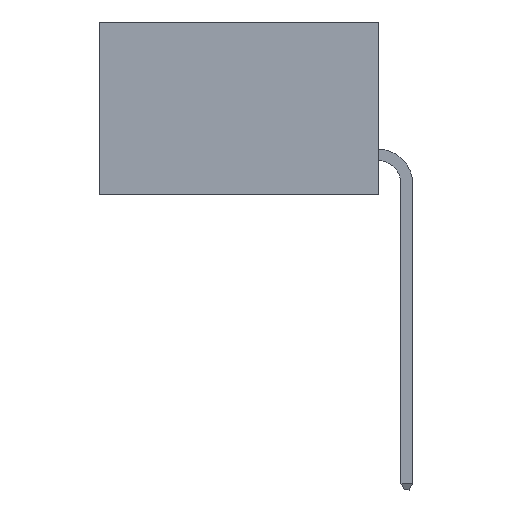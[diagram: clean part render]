
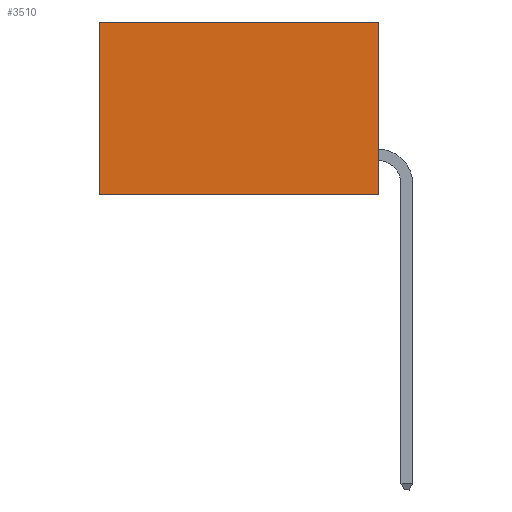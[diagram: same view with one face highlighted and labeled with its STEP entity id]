
A CAD part, left-side view. The second image highlights one B-rep face of the part: STEP entity #3510.
In plain terms, the highlighted planar face has unit normal (-1, 0, 0).
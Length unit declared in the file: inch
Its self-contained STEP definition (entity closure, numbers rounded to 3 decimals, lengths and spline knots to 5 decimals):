
#784 = LINE ( 'NONE', #14270, #11779 ) ;
#1251 = VERTEX_POINT ( 'NONE', #3374 ) ;
#1841 = CARTESIAN_POINT ( 'NONE',  ( 0.298, 0.6, 0. ) ) ;
#2229 = FACE_OUTER_BOUND ( 'NONE', #10785, .T. ) ;
#2620 = VECTOR ( 'NONE', #9039, 39.37008 ) ;
#2733 = CARTESIAN_POINT ( 'NONE',  ( 0.298, 0., 0. ) ) ;
#3042 = EDGE_CURVE ( 'NONE', #9980, #5727, #15779, .T. ) ;
#3374 = CARTESIAN_POINT ( 'NONE',  ( 0.298, 0.6, 0. ) ) ;
#3510 = ADVANCED_FACE ( 'NONE', ( #2229 ), #14328, .F. ) ;
#3634 = VECTOR ( 'NONE', #14166, 39.37008 ) ;
#4290 = ORIENTED_EDGE ( 'NONE', *, *, #15978, .T. ) ;
#5326 = EDGE_CURVE ( 'NONE', #1251, #5727, #12581, .T. ) ;
#5550 = CARTESIAN_POINT ( 'NONE',  ( 0.298, 0., -0.37 ) ) ;
#5564 = CARTESIAN_POINT ( 'NONE',  ( 0.298, 0.6, -0.37 ) ) ;
#5727 = VERTEX_POINT ( 'NONE', #5564 ) ;
#5979 = LINE ( 'NONE', #2733, #2620 ) ;
#6867 = DIRECTION ( 'NONE',  ( 1., 0., 0. ) ) ;
#6914 = DIRECTION ( 'NONE',  ( 0., 1., 0. ) ) ;
#7186 = AXIS2_PLACEMENT_3D ( 'NONE', #8000, #6867, #11705 ) ;
#7565 = ORIENTED_EDGE ( 'NONE', *, *, #3042, .F. ) ;
#8000 = CARTESIAN_POINT ( 'NONE',  ( 0.298, 0., 0. ) ) ;
#8459 = CARTESIAN_POINT ( 'NONE',  ( 0.298, 0., 0. ) ) ;
#9039 = DIRECTION ( 'NONE',  ( 0., 0., -1. ) ) ;
#9157 = CARTESIAN_POINT ( 'NONE',  ( 0.298, 0., -0.37 ) ) ;
#9980 = VERTEX_POINT ( 'NONE', #5550 ) ;
#10641 = DIRECTION ( 'NONE',  ( 0., 0., -1. ) ) ;
#10785 = EDGE_LOOP ( 'NONE', ( #11109, #7565, #15875, #4290 ) ) ;
#10839 = VECTOR ( 'NONE', #10641, 39.37008 ) ;
#11109 = ORIENTED_EDGE ( 'NONE', *, *, #5326, .T. ) ;
#11378 = EDGE_CURVE ( 'NONE', #11445, #9980, #5979, .T. ) ;
#11445 = VERTEX_POINT ( 'NONE', #8459 ) ;
#11705 = DIRECTION ( 'NONE',  ( 0., 0., -1. ) ) ;
#11779 = VECTOR ( 'NONE', #6914, 39.37008 ) ;
#12581 = LINE ( 'NONE', #1841, #10839 ) ;
#14166 = DIRECTION ( 'NONE',  ( 0., 1., 0. ) ) ;
#14270 = CARTESIAN_POINT ( 'NONE',  ( 0.298, 0., 0. ) ) ;
#14328 = PLANE ( 'NONE',  #7186 ) ;
#15779 = LINE ( 'NONE', #9157, #3634 ) ;
#15875 = ORIENTED_EDGE ( 'NONE', *, *, #11378, .F. ) ;
#15978 = EDGE_CURVE ( 'NONE', #11445, #1251, #784, .T. ) ;
